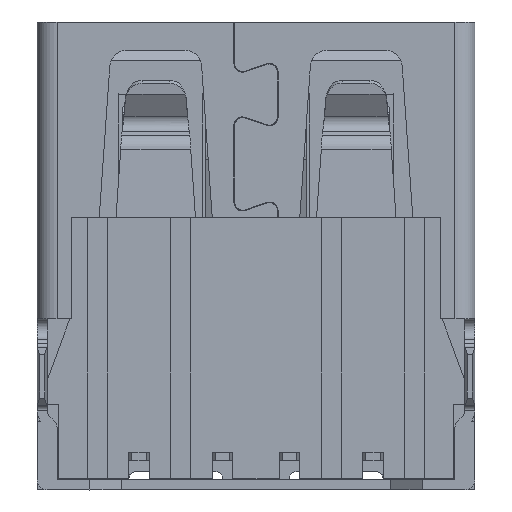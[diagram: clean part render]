
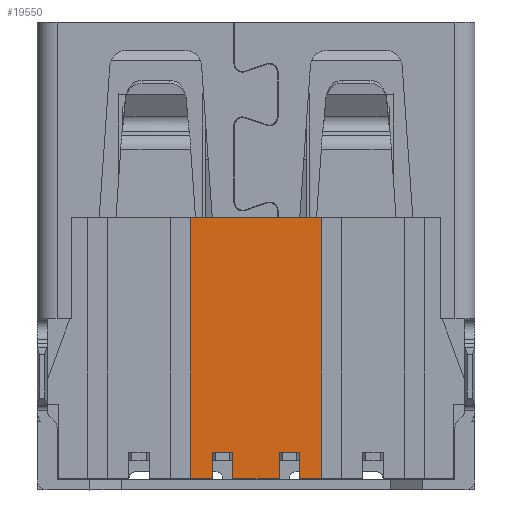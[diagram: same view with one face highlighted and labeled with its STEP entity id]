
A CAD part, front view. The second image highlights one B-rep face of the part: STEP entity #19550.
In plain terms, the highlighted planar face has unit normal (0, -1, 0).
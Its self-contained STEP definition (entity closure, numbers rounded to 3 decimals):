
#102 = CARTESIAN_POINT ( 'NONE',  ( 0., -6.1, -4.77 ) ) ;
#950 = EDGE_CURVE ( 'NONE', #27926, #24192, #7109, .T. ) ;
#1116 = CARTESIAN_POINT ( 'NONE',  ( 4.3, -6.1, 3.03 ) ) ;
#1625 = CARTESIAN_POINT ( 'NONE',  ( 0., -6.1, 0. ) ) ;
#1693 = EDGE_CURVE ( 'NONE', #7167, #7535, #27460, .T. ) ;
#1858 = DIRECTION ( 'NONE',  ( -1., 0., 0. ) ) ;
#1889 = VERTEX_POINT ( 'NONE', #4607 ) ;
#2648 = EDGE_CURVE ( 'NONE', #10158, #22150, #13407, .T. ) ;
#3980 = VECTOR ( 'NONE', #25220, 1000. ) ;
#4049 = DIRECTION ( 'NONE',  ( -1., 0., 0. ) ) ;
#4330 = DIRECTION ( 'NONE',  ( 0., 0., -1. ) ) ;
#4607 = CARTESIAN_POINT ( 'NONE',  ( 5.55, -6.1, -4.77 ) ) ;
#5227 = ORIENTED_EDGE ( 'NONE', *, *, #27750, .F. ) ;
#5661 = CARTESIAN_POINT ( 'NONE',  ( 7.55, -6.1, -3.99 ) ) ;
#6154 = CARTESIAN_POINT ( 'NONE',  ( 8.2, -6.1, 3.03 ) ) ;
#6509 = CARTESIAN_POINT ( 'NONE',  ( 0., -6.1, -4.77 ) ) ;
#6741 = CARTESIAN_POINT ( 'NONE',  ( 4.95, -6.1, -4.77 ) ) ;
#6991 = DIRECTION ( 'NONE',  ( 0., 0., 1. ) ) ;
#7084 = VECTOR ( 'NONE', #4330, 1000. ) ;
#7109 = LINE ( 'NONE', #15782, #15291 ) ;
#7167 = VERTEX_POINT ( 'NONE', #17547 ) ;
#7342 = DIRECTION ( 'NONE',  ( 1., 0., 0. ) ) ;
#7535 = VERTEX_POINT ( 'NONE', #16980 ) ;
#7563 = EDGE_CURVE ( 'NONE', #9930, #20099, #23334, .T. ) ;
#7691 = VECTOR ( 'NONE', #4049, 1000. ) ;
#7694 = CARTESIAN_POINT ( 'NONE',  ( 5.55, -6.1, -3.99 ) ) ;
#8136 = CARTESIAN_POINT ( 'NONE',  ( 4.95, -6.1, -4.77 ) ) ;
#8319 = CARTESIAN_POINT ( 'NONE',  ( 7.55, -6.1, -3.99 ) ) ;
#8643 = LINE ( 'NONE', #6509, #23943 ) ;
#8751 = DIRECTION ( 'NONE',  ( 0., 0., 1. ) ) ;
#8811 = CARTESIAN_POINT ( 'NONE',  ( 4.3, -6.1, -4.77 ) ) ;
#8857 = CARTESIAN_POINT ( 'NONE',  ( 6.95, -6.1, -4.77 ) ) ;
#9930 = VERTEX_POINT ( 'NONE', #21508 ) ;
#10158 = VERTEX_POINT ( 'NONE', #16826 ) ;
#10903 = LINE ( 'NONE', #8136, #24338 ) ;
#10992 = LINE ( 'NONE', #25586, #14250 ) ;
#11615 = CARTESIAN_POINT ( 'NONE',  ( 0., -6.1, 3.03 ) ) ;
#11735 = EDGE_LOOP ( 'NONE', ( #15924, #23556, #20336, #14570, #26600, #18131, #23612, #5227, #17998, #13600, #17533, #22470 ) ) ;
#12253 = DIRECTION ( 'NONE',  ( 0., 0., -1. ) ) ;
#12432 = EDGE_CURVE ( 'NONE', #22150, #15763, #10992, .T. ) ;
#13407 = LINE ( 'NONE', #8857, #13554 ) ;
#13554 = VECTOR ( 'NONE', #6991, 1000. ) ;
#13600 = ORIENTED_EDGE ( 'NONE', *, *, #1693, .T. ) ;
#13771 = AXIS2_PLACEMENT_3D ( 'NONE', #1625, #21181, #21324 ) ;
#13844 = VERTEX_POINT ( 'NONE', #6741 ) ;
#14250 = VECTOR ( 'NONE', #21477, 1000. ) ;
#14570 = ORIENTED_EDGE ( 'NONE', *, *, #7563, .F. ) ;
#14715 = LINE ( 'NONE', #8319, #7084 ) ;
#15291 = VECTOR ( 'NONE', #24420, 1000. ) ;
#15763 = VERTEX_POINT ( 'NONE', #5661 ) ;
#15782 = CARTESIAN_POINT ( 'NONE',  ( 4.3, -6.1, 0. ) ) ;
#15837 = VECTOR ( 'NONE', #7342, 1000. ) ;
#15924 = ORIENTED_EDGE ( 'NONE', *, *, #2648, .T. ) ;
#16228 = EDGE_CURVE ( 'NONE', #15763, #20099, #14715, .T. ) ;
#16633 = VERTEX_POINT ( 'NONE', #6154 ) ;
#16738 = CARTESIAN_POINT ( 'NONE',  ( 8.2, -6.1, 0. ) ) ;
#16826 = CARTESIAN_POINT ( 'NONE',  ( 6.95, -6.1, -4.77 ) ) ;
#16876 = EDGE_CURVE ( 'NONE', #9930, #16633, #20833, .T. ) ;
#16980 = CARTESIAN_POINT ( 'NONE',  ( 5.55, -6.1, -3.99 ) ) ;
#17451 = CARTESIAN_POINT ( 'NONE',  ( 7.55, -6.1, -4.77 ) ) ;
#17533 = ORIENTED_EDGE ( 'NONE', *, *, #26373, .T. ) ;
#17547 = CARTESIAN_POINT ( 'NONE',  ( 4.95, -6.1, -3.99 ) ) ;
#17998 = ORIENTED_EDGE ( 'NONE', *, *, #18990, .T. ) ;
#18131 = ORIENTED_EDGE ( 'NONE', *, *, #24623, .F. ) ;
#18990 = EDGE_CURVE ( 'NONE', #13844, #7167, #10903, .T. ) ;
#19550 = ADVANCED_FACE ( 'NONE', ( #21461 ), #23301, .T. ) ;
#19589 = VECTOR ( 'NONE', #25738, 1000. ) ;
#20099 = VERTEX_POINT ( 'NONE', #17451 ) ;
#20292 = VECTOR ( 'NONE', #25194, 1000. ) ;
#20336 = ORIENTED_EDGE ( 'NONE', *, *, #16228, .T. ) ;
#20375 = CARTESIAN_POINT ( 'NONE',  ( 0., -6.1, -3.99 ) ) ;
#20833 = LINE ( 'NONE', #16738, #3980 ) ;
#21181 = DIRECTION ( 'NONE',  ( 0., -1., 0. ) ) ;
#21324 = DIRECTION ( 'NONE',  ( -1., 0., 0. ) ) ;
#21461 = FACE_OUTER_BOUND ( 'NONE', #11735, .T. ) ;
#21477 = DIRECTION ( 'NONE',  ( 1., 0., 0. ) ) ;
#21508 = CARTESIAN_POINT ( 'NONE',  ( 8.2, -6.1, -4.77 ) ) ;
#22150 = VERTEX_POINT ( 'NONE', #27482 ) ;
#22470 = ORIENTED_EDGE ( 'NONE', *, *, #23852, .F. ) ;
#23301 = PLANE ( 'NONE',  #13771 ) ;
#23334 = LINE ( 'NONE', #102, #19589 ) ;
#23556 = ORIENTED_EDGE ( 'NONE', *, *, #12432, .T. ) ;
#23612 = ORIENTED_EDGE ( 'NONE', *, *, #950, .T. ) ;
#23852 = EDGE_CURVE ( 'NONE', #10158, #1889, #27728, .T. ) ;
#23943 = VECTOR ( 'NONE', #1858, 1000. ) ;
#24192 = VERTEX_POINT ( 'NONE', #8811 ) ;
#24338 = VECTOR ( 'NONE', #8751, 1000. ) ;
#24345 = VECTOR ( 'NONE', #12253, 1000. ) ;
#24420 = DIRECTION ( 'NONE',  ( 0., 0., -1. ) ) ;
#24623 = EDGE_CURVE ( 'NONE', #27926, #16633, #26772, .T. ) ;
#25194 = DIRECTION ( 'NONE',  ( 1., 0., 0. ) ) ;
#25220 = DIRECTION ( 'NONE',  ( 0., 0., 1. ) ) ;
#25586 = CARTESIAN_POINT ( 'NONE',  ( 0., -6.1, -3.99 ) ) ;
#25738 = DIRECTION ( 'NONE',  ( -1., 0., 0. ) ) ;
#26373 = EDGE_CURVE ( 'NONE', #7535, #1889, #27393, .T. ) ;
#26600 = ORIENTED_EDGE ( 'NONE', *, *, #16876, .T. ) ;
#26772 = LINE ( 'NONE', #11615, #15837 ) ;
#27296 = CARTESIAN_POINT ( 'NONE',  ( 0., -6.1, -4.77 ) ) ;
#27393 = LINE ( 'NONE', #7694, #24345 ) ;
#27460 = LINE ( 'NONE', #20375, #20292 ) ;
#27482 = CARTESIAN_POINT ( 'NONE',  ( 6.95, -6.1, -3.99 ) ) ;
#27728 = LINE ( 'NONE', #27296, #7691 ) ;
#27750 = EDGE_CURVE ( 'NONE', #13844, #24192, #8643, .T. ) ;
#27926 = VERTEX_POINT ( 'NONE', #1116 ) ;
